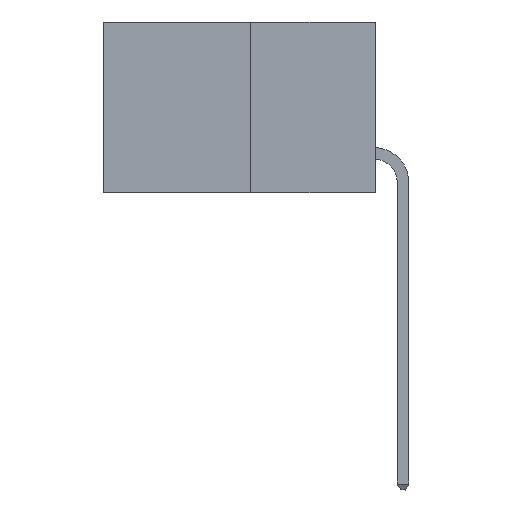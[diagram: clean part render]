
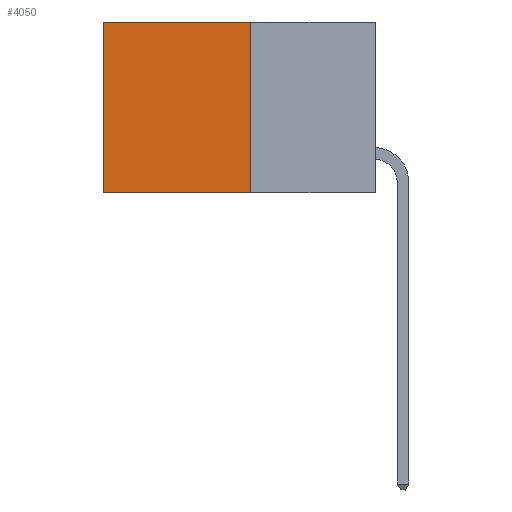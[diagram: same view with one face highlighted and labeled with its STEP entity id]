
A CAD part, left-side view. The second image highlights one B-rep face of the part: STEP entity #4050.
In plain terms, the highlighted planar face has unit normal (-1, 0, 0).
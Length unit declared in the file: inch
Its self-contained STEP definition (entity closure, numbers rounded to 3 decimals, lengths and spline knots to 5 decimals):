
#335 = LINE ( 'NONE', #16055, #10680 ) ;
#392 = EDGE_CURVE ( 'NONE', #4464, #12075, #11959, .T. ) ;
#1090 = CARTESIAN_POINT ( 'NONE',  ( 0.277, 0.59, -0.37 ) ) ;
#1156 = ORIENTED_EDGE ( 'NONE', *, *, #5679, .F. ) ;
#1407 = CARTESIAN_POINT ( 'NONE',  ( 0.277, 0.27, 0. ) ) ;
#1999 = DIRECTION ( 'NONE',  ( 0., 1., 0. ) ) ;
#2147 = DIRECTION ( 'NONE',  ( 1., 0., 0. ) ) ;
#2886 = VERTEX_POINT ( 'NONE', #1407 ) ;
#2893 = EDGE_CURVE ( 'NONE', #6286, #12075, #10467, .T. ) ;
#3188 = EDGE_LOOP ( 'NONE', ( #6744, #14915, #1156, #17619 ) ) ;
#3793 = CARTESIAN_POINT ( 'NONE',  ( 0.277, 0.59, -0.37 ) ) ;
#3994 = VECTOR ( 'NONE', #1999, 39.37008 ) ;
#4050 = ADVANCED_FACE ( 'NONE', ( #13474 ), #10626, .F. ) ;
#4464 = VERTEX_POINT ( 'NONE', #5835 ) ;
#4907 = CARTESIAN_POINT ( 'NONE',  ( 0.277, 0.27, -0.37 ) ) ;
#5662 = CARTESIAN_POINT ( 'NONE',  ( 0.277, 0.59, 0. ) ) ;
#5679 = EDGE_CURVE ( 'NONE', #2886, #4464, #16028, .T. ) ;
#5835 = CARTESIAN_POINT ( 'NONE',  ( 0.277, 0.27, -0.37 ) ) ;
#6286 = VERTEX_POINT ( 'NONE', #5662 ) ;
#6744 = ORIENTED_EDGE ( 'NONE', *, *, #2893, .T. ) ;
#7699 = VECTOR ( 'NONE', #11592, 39.37008 ) ;
#8775 = CARTESIAN_POINT ( 'NONE',  ( 0.277, 0.27, -0.37 ) ) ;
#10467 = LINE ( 'NONE', #3793, #17458 ) ;
#10626 = PLANE ( 'NONE',  #15165 ) ;
#10680 = VECTOR ( 'NONE', #17473, 39.37008 ) ;
#10730 = EDGE_CURVE ( 'NONE', #2886, #6286, #335, .T. ) ;
#11592 = DIRECTION ( 'NONE',  ( 0., 0., -1. ) ) ;
#11959 = LINE ( 'NONE', #13845, #3994 ) ;
#12009 = DIRECTION ( 'NONE',  ( 0., 0., -1. ) ) ;
#12075 = VERTEX_POINT ( 'NONE', #1090 ) ;
#13474 = FACE_OUTER_BOUND ( 'NONE', #3188, .T. ) ;
#13845 = CARTESIAN_POINT ( 'NONE',  ( 0.277, 0.27, -0.37 ) ) ;
#14915 = ORIENTED_EDGE ( 'NONE', *, *, #392, .F. ) ;
#15165 = AXIS2_PLACEMENT_3D ( 'NONE', #4907, #2147, #12009 ) ;
#15386 = DIRECTION ( 'NONE',  ( 0., 0., -1. ) ) ;
#16028 = LINE ( 'NONE', #8775, #7699 ) ;
#16055 = CARTESIAN_POINT ( 'NONE',  ( 0.277, 0.27, 0. ) ) ;
#17458 = VECTOR ( 'NONE', #15386, 39.37008 ) ;
#17473 = DIRECTION ( 'NONE',  ( 0., 1., 0. ) ) ;
#17619 = ORIENTED_EDGE ( 'NONE', *, *, #10730, .T. ) ;
